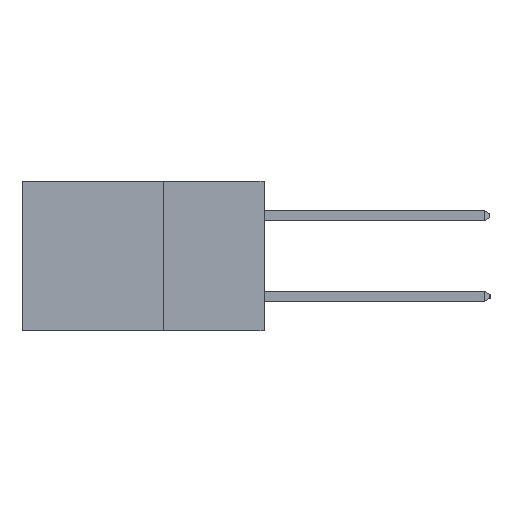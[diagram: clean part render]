
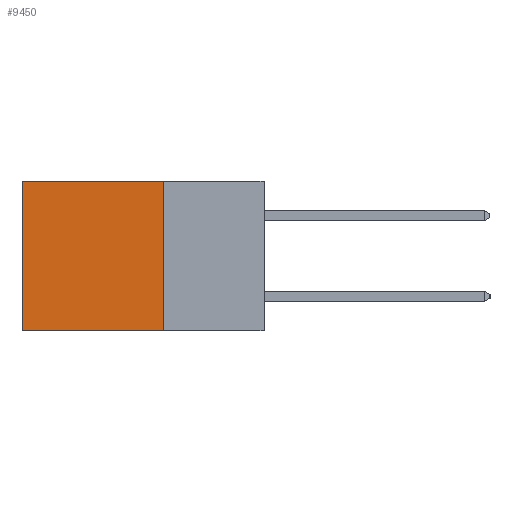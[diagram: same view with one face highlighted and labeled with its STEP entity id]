
A CAD part, left-side view. The second image highlights one B-rep face of the part: STEP entity #9450.
In plain terms, the highlighted planar face has unit normal (-1, 0, 0).
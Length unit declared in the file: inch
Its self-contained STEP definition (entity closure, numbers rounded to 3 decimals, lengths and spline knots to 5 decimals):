
#598 = VECTOR ( 'NONE', #23302, 39.37008 ) ;
#1262 = DIRECTION ( 'NONE',  ( 1., 0., 0. ) ) ;
#1908 = LINE ( 'NONE', #23392, #598 ) ;
#2267 = FACE_OUTER_BOUND ( 'NONE', #16094, .T. ) ;
#3092 = VECTOR ( 'NONE', #20047, 39.37008 ) ;
#3719 = LINE ( 'NONE', #21353, #3092 ) ;
#4258 = EDGE_CURVE ( 'NONE', #21769, #8362, #1908, .T. ) ;
#4457 = VERTEX_POINT ( 'NONE', #20405 ) ;
#5226 = PLANE ( 'NONE',  #15355 ) ;
#6190 = EDGE_CURVE ( 'NONE', #4457, #8362, #3719, .T. ) ;
#6320 = EDGE_CURVE ( 'NONE', #15171, #21769, #15863, .T. ) ;
#6413 = VECTOR ( 'NONE', #11435, 39.37008 ) ;
#7666 = CARTESIAN_POINT ( 'NONE',  ( 0.2615, 0.25, 0. ) ) ;
#8362 = VERTEX_POINT ( 'NONE', #20053 ) ;
#8724 = DIRECTION ( 'NONE',  ( 0., 1., 0. ) ) ;
#9208 = ORIENTED_EDGE ( 'NONE', *, *, #23897, .F. ) ;
#9450 = ADVANCED_FACE ( 'NONE', ( #2267 ), #5226, .F. ) ;
#11435 = DIRECTION ( 'NONE',  ( 0., 0., -1. ) ) ;
#11729 = LINE ( 'NONE', #19210, #6413 ) ;
#15171 = VERTEX_POINT ( 'NONE', #21941 ) ;
#15277 = DIRECTION ( 'NONE',  ( 0., 0., -1. ) ) ;
#15355 = AXIS2_PLACEMENT_3D ( 'NONE', #21030, #1262, #15277 ) ;
#15863 = LINE ( 'NONE', #7666, #21009 ) ;
#15960 = ORIENTED_EDGE ( 'NONE', *, *, #4258, .T. ) ;
#16094 = EDGE_LOOP ( 'NONE', ( #15960, #22203, #9208, #19193 ) ) ;
#19193 = ORIENTED_EDGE ( 'NONE', *, *, #6320, .T. ) ;
#19210 = CARTESIAN_POINT ( 'NONE',  ( 0.2615, 0.25, -0.37 ) ) ;
#20047 = DIRECTION ( 'NONE',  ( 0., 1., 0. ) ) ;
#20053 = CARTESIAN_POINT ( 'NONE',  ( 0.2615, 0.6, -0.37 ) ) ;
#20405 = CARTESIAN_POINT ( 'NONE',  ( 0.2615, 0.25, -0.37 ) ) ;
#21009 = VECTOR ( 'NONE', #8724, 39.37008 ) ;
#21030 = CARTESIAN_POINT ( 'NONE',  ( 0.2615, 0.25, -0.37 ) ) ;
#21353 = CARTESIAN_POINT ( 'NONE',  ( 0.2615, 0.25, -0.37 ) ) ;
#21769 = VERTEX_POINT ( 'NONE', #22864 ) ;
#21941 = CARTESIAN_POINT ( 'NONE',  ( 0.2615, 0.25, 0. ) ) ;
#22203 = ORIENTED_EDGE ( 'NONE', *, *, #6190, .F. ) ;
#22864 = CARTESIAN_POINT ( 'NONE',  ( 0.2615, 0.6, 0. ) ) ;
#23302 = DIRECTION ( 'NONE',  ( 0., 0., -1. ) ) ;
#23392 = CARTESIAN_POINT ( 'NONE',  ( 0.2615, 0.6, -0.37 ) ) ;
#23897 = EDGE_CURVE ( 'NONE', #15171, #4457, #11729, .T. ) ;
